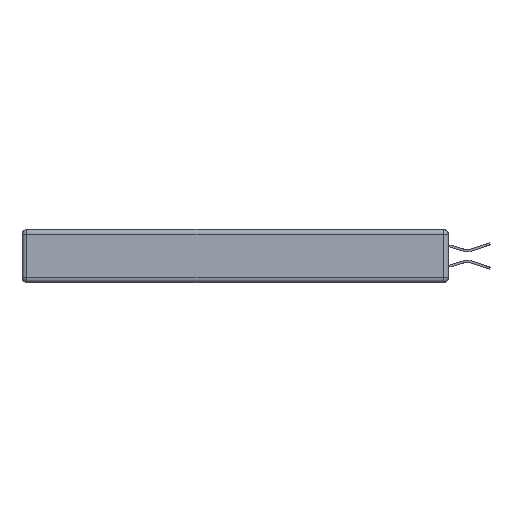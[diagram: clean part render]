
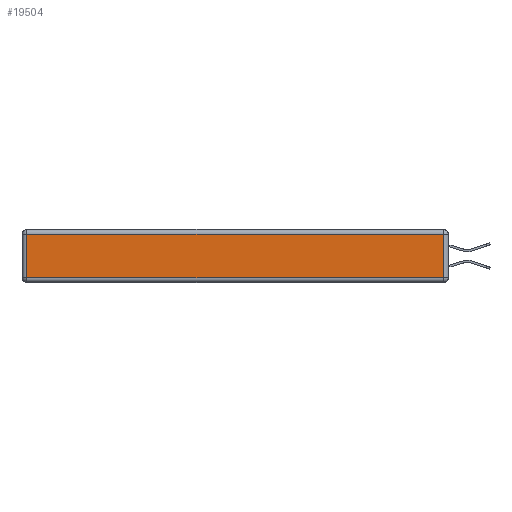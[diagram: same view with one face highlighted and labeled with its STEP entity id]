
A CAD part, left-side view. The second image highlights one B-rep face of the part: STEP entity #19504.
In plain terms, the highlighted planar face has unit normal (-1, 0, 0).
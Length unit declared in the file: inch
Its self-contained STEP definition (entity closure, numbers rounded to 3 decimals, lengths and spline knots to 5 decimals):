
#2851 = VECTOR ( 'NONE', #4944, 39.37008 ) ;
#3082 = EDGE_CURVE ( 'NONE', #7700, #7748, #5225, .T. ) ;
#3838 = FACE_OUTER_BOUND ( 'NONE', #4528, .T. ) ;
#4492 = VECTOR ( 'NONE', #20439, 39.37008 ) ;
#4528 = EDGE_LOOP ( 'NONE', ( #12062, #15459, #12794, #28982 ) ) ;
#4554 = VERTEX_POINT ( 'NONE', #19909 ) ;
#4693 = LINE ( 'NONE', #24115, #17284 ) ;
#4944 = DIRECTION ( 'NONE',  ( 0., 1., 0. ) ) ;
#5225 = LINE ( 'NONE', #22134, #2851 ) ;
#5544 = DIRECTION ( 'NONE',  ( -1., 0., 0. ) ) ;
#7700 = VERTEX_POINT ( 'NONE', #14267 ) ;
#7748 = VERTEX_POINT ( 'NONE', #29911 ) ;
#8686 = EDGE_CURVE ( 'NONE', #10015, #7700, #4693, .T. ) ;
#9041 = VECTOR ( 'NONE', #9245, 39.37008 ) ;
#9245 = DIRECTION ( 'NONE',  ( 0., -1., 0. ) ) ;
#10015 = VERTEX_POINT ( 'NONE', #28539 ) ;
#12062 = ORIENTED_EDGE ( 'NONE', *, *, #16157, .T. ) ;
#12338 = LINE ( 'NONE', #12813, #4492 ) ;
#12794 = ORIENTED_EDGE ( 'NONE', *, *, #3082, .T. ) ;
#12813 = CARTESIAN_POINT ( 'NONE',  ( 0., 2.72, -0.343 ) ) ;
#13014 = CARTESIAN_POINT ( 'NONE',  ( 0., 0., -0.343 ) ) ;
#14267 = CARTESIAN_POINT ( 'NONE',  ( 0., 0.03, -0.03 ) ) ;
#14460 = EDGE_CURVE ( 'NONE', #7748, #4554, #12338, .T. ) ;
#15459 = ORIENTED_EDGE ( 'NONE', *, *, #8686, .T. ) ;
#16157 = EDGE_CURVE ( 'NONE', #4554, #10015, #24029, .T. ) ;
#16759 = DIRECTION ( 'NONE',  ( 0., 0., 1. ) ) ;
#16984 = CARTESIAN_POINT ( 'NONE',  ( 0., 0., -0.313 ) ) ;
#17284 = VECTOR ( 'NONE', #16759, 39.37008 ) ;
#18801 = AXIS2_PLACEMENT_3D ( 'NONE', #13014, #5544, #24612 ) ;
#19504 = ADVANCED_FACE ( 'NONE', ( #3838 ), #25458, .T. ) ;
#19909 = CARTESIAN_POINT ( 'NONE',  ( 0., 2.72, -0.313 ) ) ;
#20439 = DIRECTION ( 'NONE',  ( 0., 0., -1. ) ) ;
#22134 = CARTESIAN_POINT ( 'NONE',  ( 0., 2.75, -0.03 ) ) ;
#24029 = LINE ( 'NONE', #16984, #9041 ) ;
#24115 = CARTESIAN_POINT ( 'NONE',  ( 0., 0.03, -0.343 ) ) ;
#24612 = DIRECTION ( 'NONE',  ( 0., 0., 1. ) ) ;
#25458 = PLANE ( 'NONE',  #18801 ) ;
#28539 = CARTESIAN_POINT ( 'NONE',  ( 0., 0.03, -0.313 ) ) ;
#28982 = ORIENTED_EDGE ( 'NONE', *, *, #14460, .T. ) ;
#29911 = CARTESIAN_POINT ( 'NONE',  ( 0., 2.72, -0.03 ) ) ;
